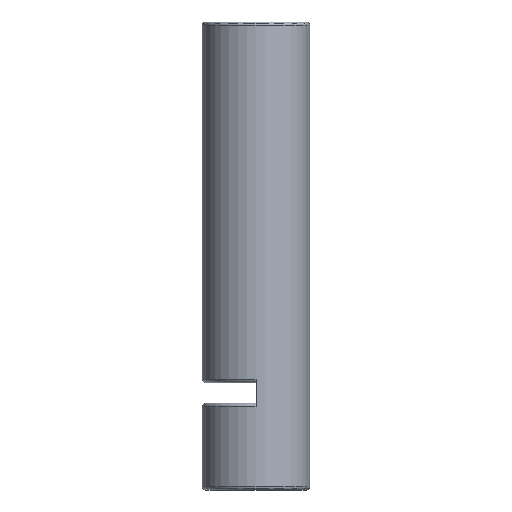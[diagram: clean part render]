
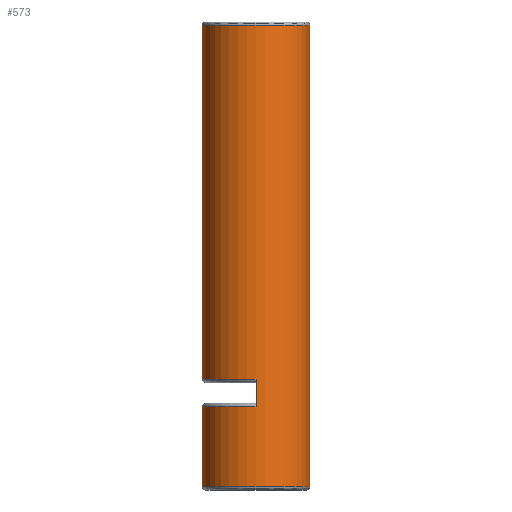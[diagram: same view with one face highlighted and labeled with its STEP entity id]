
A CAD part, front view. The second image highlights one B-rep face of the part: STEP entity #573.
In plain terms, the highlighted cylindrical face has radius 1.981 mm (diameter 3.962 mm), a partial arc.
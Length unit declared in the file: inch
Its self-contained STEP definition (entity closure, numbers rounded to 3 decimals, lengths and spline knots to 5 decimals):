
#28=DIRECTION('',(0.,0.,1.));
#29=VECTOR('',#28,0.67);
#30=CARTESIAN_POINT('',(0.078,0.,0.005));
#31=LINE('',#30,#29);
#35=DIRECTION('',(0.,0.,1.));
#36=VECTOR('',#35,0.514);
#37=CARTESIAN_POINT('',(-0.078,0.,0.161));
#38=LINE('',#37,#36);
#49=DIRECTION('',(0.,0.,1.));
#50=VECTOR('',#49,0.116);
#51=CARTESIAN_POINT('',(-0.078,0.,0.005));
#52=LINE('',#51,#50);
#64=CARTESIAN_POINT('',(0.,0.,0.005));
#65=DIRECTION('',(0.,0.,-1.));
#66=DIRECTION('',(1.,0.,0.));
#67=AXIS2_PLACEMENT_3D('',#64,#65,#66);
#88=DIRECTION('',(0.,0.,-1.));
#89=VECTOR('',#88,0.04);
#90=CARTESIAN_POINT('',(0.,-0.078,0.161));
#91=LINE('',#90,#89);
#95=CARTESIAN_POINT('',(0.,0.,0.121));
#96=DIRECTION('',(0.,0.,1.));
#97=DIRECTION('',(-1.,0.,0.));
#98=AXIS2_PLACEMENT_3D('',#95,#96,#97);
#321=CARTESIAN_POINT('',(0.,0.,0.675));
#322=DIRECTION('',(0.,0.,1.));
#323=DIRECTION('',(-1.,0.,0.));
#324=AXIS2_PLACEMENT_3D('',#321,#322,#323);
#414=CARTESIAN_POINT('',(0.,0.,0.161));
#415=DIRECTION('',(0.,0.,-1.));
#416=DIRECTION('',(0.,-1.,0.));
#417=AXIS2_PLACEMENT_3D('',#414,#415,#416);
#423=CARTESIAN_POINT('',(0.,-0.078,0.121));
#425=VERTEX_POINT('',#423);
#440=CARTESIAN_POINT('',(0.,-0.078,0.161));
#441=VERTEX_POINT('',#440);
#446=CARTESIAN_POINT('',(0.078,0.,0.675));
#448=VERTEX_POINT('',#446);
#452=CARTESIAN_POINT('',(-0.078,0.,0.675));
#453=VERTEX_POINT('',#452);
#458=CARTESIAN_POINT('',(-0.078,0.,0.005));
#459=CARTESIAN_POINT('',(-0.078,0.,0.121));
#460=VERTEX_POINT('',#458);
#461=VERTEX_POINT('',#459);
#462=CARTESIAN_POINT('',(-0.078,0.,0.161));
#463=VERTEX_POINT('',#462);
#464=CARTESIAN_POINT('',(0.078,0.,0.005));
#465=VERTEX_POINT('',#464);
#554=CARTESIAN_POINT('',(0.,0.,0.));
#555=DIRECTION('',(0.,0.,1.));
#556=DIRECTION('',(-1.,0.,0.));
#557=AXIS2_PLACEMENT_3D('',#554,#555,#556);
#558=CYLINDRICAL_SURFACE('',#557,0.078);
#559=ORIENTED_EDGE('',*,*,#545,.T.);
#560=ORIENTED_EDGE('',*,*,#520,.T.);
#562=ORIENTED_EDGE('',*,*,#561,.T.);
#564=ORIENTED_EDGE('',*,*,#563,.F.);
#566=ORIENTED_EDGE('',*,*,#565,.T.);
#567=ORIENTED_EDGE('',*,*,#512,.T.);
#569=ORIENTED_EDGE('',*,*,#568,.T.);
#570=ORIENTED_EDGE('',*,*,#509,.F.);
#571=EDGE_LOOP('',(#559,#560,#562,#564,#566,#567,#569,#570));
#572=FACE_OUTER_BOUND('',#571,.F.);
#68=CIRCLE('',#67,0.078);
#99=CIRCLE('',#98,0.078);
#325=CIRCLE('',#324,0.078);
#418=CIRCLE('',#417,0.078);
#509=EDGE_CURVE('',#465,#448,#31,.T.);
#512=EDGE_CURVE('',#463,#453,#38,.T.);
#520=EDGE_CURVE('',#460,#461,#52,.T.);
#545=EDGE_CURVE('',#465,#460,#68,.T.);
#561=EDGE_CURVE('',#461,#425,#99,.T.);
#563=EDGE_CURVE('',#441,#425,#91,.T.);
#565=EDGE_CURVE('',#441,#463,#418,.T.);
#568=EDGE_CURVE('',#453,#448,#325,.T.);
#573=ADVANCED_FACE('',(#572),#558,.T.);
